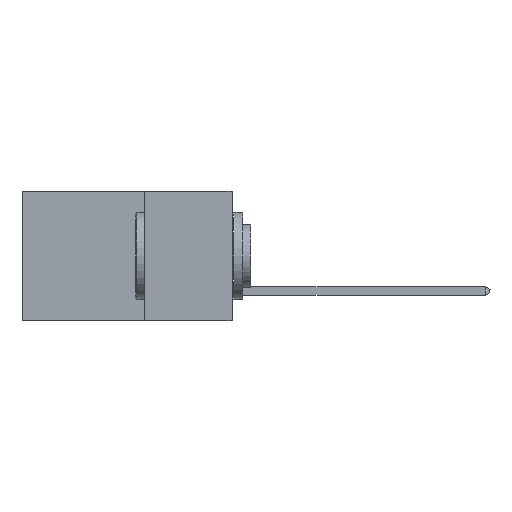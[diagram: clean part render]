
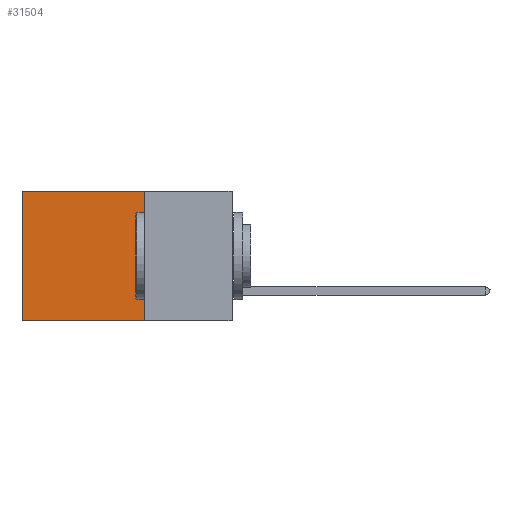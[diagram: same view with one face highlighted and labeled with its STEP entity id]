
A CAD part, left-side view. The second image highlights one B-rep face of the part: STEP entity #31504.
In plain terms, the highlighted planar face has unit normal (-1, 0, 0).
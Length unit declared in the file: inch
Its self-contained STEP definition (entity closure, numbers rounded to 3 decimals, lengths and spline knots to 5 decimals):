
#1446 = VECTOR ( 'NONE', #36686, 39.37008 ) ;
#1679 = ORIENTED_EDGE ( 'NONE', *, *, #21155, .T. ) ;
#2092 = VERTEX_POINT ( 'NONE', #47008 ) ;
#2501 = VERTEX_POINT ( 'NONE', #26795 ) ;
#3764 = ORIENTED_EDGE ( 'NONE', *, *, #29615, .F. ) ;
#3902 = DIRECTION ( 'NONE',  ( 0., 0., -1. ) ) ;
#4309 = CARTESIAN_POINT ( 'NONE',  ( 0.2875, 0.25, 0. ) ) ;
#6749 = CARTESIAN_POINT ( 'NONE',  ( 0.2875, 0.6, 0. ) ) ;
#9944 = CARTESIAN_POINT ( 'NONE',  ( 0.2875, 0.25, -0.37 ) ) ;
#10423 = DIRECTION ( 'NONE',  ( 0., 0., -1. ) ) ;
#10663 = EDGE_LOOP ( 'NONE', ( #40624, #3764, #28319, #1679 ) ) ;
#12064 = DIRECTION ( 'NONE',  ( 1., 0., 0. ) ) ;
#15825 = EDGE_CURVE ( 'NONE', #2092, #2501, #33350, .T. ) ;
#16134 = LINE ( 'NONE', #39908, #38240 ) ;
#16871 = FACE_OUTER_BOUND ( 'NONE', #10663, .T. ) ;
#18471 = LINE ( 'NONE', #9944, #1446 ) ;
#20437 = VECTOR ( 'NONE', #31795, 39.37008 ) ;
#21155 = EDGE_CURVE ( 'NONE', #28854, #2092, #45660, .T. ) ;
#26511 = AXIS2_PLACEMENT_3D ( 'NONE', #4309, #12064, #46581 ) ;
#26795 = CARTESIAN_POINT ( 'NONE',  ( 0.2875, 0.6, -0.37 ) ) ;
#28275 = PLANE ( 'NONE',  #26511 ) ;
#28319 = ORIENTED_EDGE ( 'NONE', *, *, #33706, .F. ) ;
#28854 = VERTEX_POINT ( 'NONE', #35761 ) ;
#29615 = EDGE_CURVE ( 'NONE', #47632, #2501, #18471, .T. ) ;
#31504 = ADVANCED_FACE ( 'NONE', ( #16871 ), #28275, .F. ) ;
#31795 = DIRECTION ( 'NONE',  ( 0., 1., 0. ) ) ;
#33350 = LINE ( 'NONE', #6749, #45890 ) ;
#33706 = EDGE_CURVE ( 'NONE', #28854, #47632, #16134, .T. ) ;
#35629 = CARTESIAN_POINT ( 'NONE',  ( 0.2875, 0.25, 0. ) ) ;
#35761 = CARTESIAN_POINT ( 'NONE',  ( 0.2875, 0.25, 0. ) ) ;
#36686 = DIRECTION ( 'NONE',  ( 0., 1., 0. ) ) ;
#38097 = CARTESIAN_POINT ( 'NONE',  ( 0.2875, 0.25, -0.37 ) ) ;
#38240 = VECTOR ( 'NONE', #3902, 39.37008 ) ;
#39908 = CARTESIAN_POINT ( 'NONE',  ( 0.2875, 0.25, 0. ) ) ;
#40624 = ORIENTED_EDGE ( 'NONE', *, *, #15825, .T. ) ;
#45660 = LINE ( 'NONE', #35629, #20437 ) ;
#45890 = VECTOR ( 'NONE', #10423, 39.37008 ) ;
#46581 = DIRECTION ( 'NONE',  ( 0., 0., -1. ) ) ;
#47008 = CARTESIAN_POINT ( 'NONE',  ( 0.2875, 0.6, 0. ) ) ;
#47632 = VERTEX_POINT ( 'NONE', #38097 ) ;
